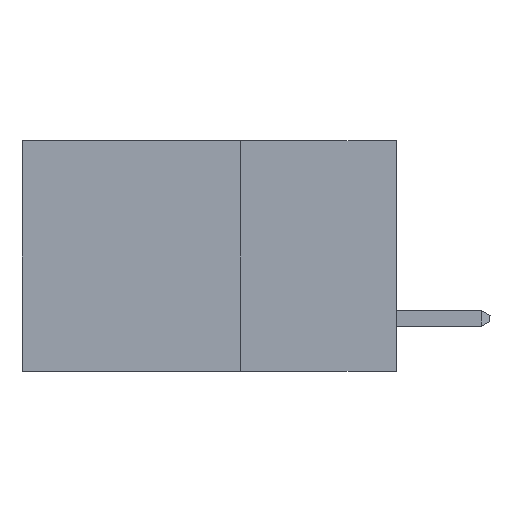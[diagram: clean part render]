
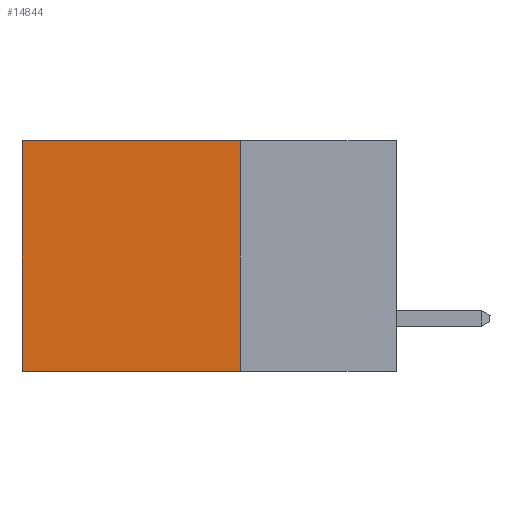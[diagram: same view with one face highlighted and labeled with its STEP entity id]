
A CAD part, left-side view. The second image highlights one B-rep face of the part: STEP entity #14844.
In plain terms, the highlighted planar face has unit normal (-1, 0, 0).
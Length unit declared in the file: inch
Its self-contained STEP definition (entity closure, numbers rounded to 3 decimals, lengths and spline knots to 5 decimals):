
#186 = CARTESIAN_POINT ( 'NONE',  ( 0.2615, 0.25, -0.37 ) ) ;
#282 = ORIENTED_EDGE ( 'NONE', *, *, #9038, .F. ) ;
#943 = DIRECTION ( 'NONE',  ( 1., 0., 0. ) ) ;
#1877 = ORIENTED_EDGE ( 'NONE', *, *, #4596, .T. ) ;
#1924 = DIRECTION ( 'NONE',  ( 0., 0., -1. ) ) ;
#2749 = LINE ( 'NONE', #186, #12437 ) ;
#3253 = CARTESIAN_POINT ( 'NONE',  ( 0.2615, 0.25, -0.37 ) ) ;
#3376 = LINE ( 'NONE', #8812, #6170 ) ;
#3465 = EDGE_CURVE ( 'NONE', #13225, #16947, #9074, .T. ) ;
#4025 = VECTOR ( 'NONE', #16001, 39.37008 ) ;
#4574 = CARTESIAN_POINT ( 'NONE',  ( 0.2615, 0.25, 0. ) ) ;
#4596 = EDGE_CURVE ( 'NONE', #10630, #13225, #3376, .T. ) ;
#4919 = CARTESIAN_POINT ( 'NONE',  ( 0.2615, 0.6, -0.37 ) ) ;
#5387 = VECTOR ( 'NONE', #10748, 39.37008 ) ;
#6170 = VECTOR ( 'NONE', #6363, 39.37008 ) ;
#6363 = DIRECTION ( 'NONE',  ( 0., 1., 0. ) ) ;
#6385 = CARTESIAN_POINT ( 'NONE',  ( 0.2615, 0.25, -0.37 ) ) ;
#6734 = LINE ( 'NONE', #12103, #5387 ) ;
#7303 = VERTEX_POINT ( 'NONE', #6385 ) ;
#7495 = AXIS2_PLACEMENT_3D ( 'NONE', #3253, #943, #1924 ) ;
#8008 = ORIENTED_EDGE ( 'NONE', *, *, #3465, .T. ) ;
#8168 = EDGE_CURVE ( 'NONE', #7303, #16947, #6734, .T. ) ;
#8436 = DIRECTION ( 'NONE',  ( 0., 0., -1. ) ) ;
#8812 = CARTESIAN_POINT ( 'NONE',  ( 0.2615, 0.25, 0. ) ) ;
#9038 = EDGE_CURVE ( 'NONE', #10630, #7303, #2749, .T. ) ;
#9074 = LINE ( 'NONE', #4919, #4025 ) ;
#9524 = CARTESIAN_POINT ( 'NONE',  ( 0.2615, 0.6, 0. ) ) ;
#10630 = VERTEX_POINT ( 'NONE', #4574 ) ;
#10748 = DIRECTION ( 'NONE',  ( 0., 1., 0. ) ) ;
#11766 = PLANE ( 'NONE',  #7495 ) ;
#12103 = CARTESIAN_POINT ( 'NONE',  ( 0.2615, 0.25, -0.37 ) ) ;
#12437 = VECTOR ( 'NONE', #8436, 39.37008 ) ;
#13208 = ORIENTED_EDGE ( 'NONE', *, *, #8168, .F. ) ;
#13225 = VERTEX_POINT ( 'NONE', #9524 ) ;
#14844 = ADVANCED_FACE ( 'NONE', ( #15431 ), #11766, .F. ) ;
#15389 = CARTESIAN_POINT ( 'NONE',  ( 0.2615, 0.6, -0.37 ) ) ;
#15431 = FACE_OUTER_BOUND ( 'NONE', #15713, .T. ) ;
#15713 = EDGE_LOOP ( 'NONE', ( #8008, #13208, #282, #1877 ) ) ;
#16001 = DIRECTION ( 'NONE',  ( 0., 0., -1. ) ) ;
#16947 = VERTEX_POINT ( 'NONE', #15389 ) ;
